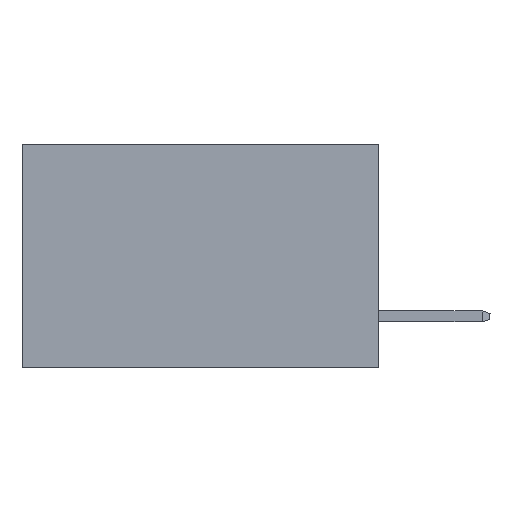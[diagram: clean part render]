
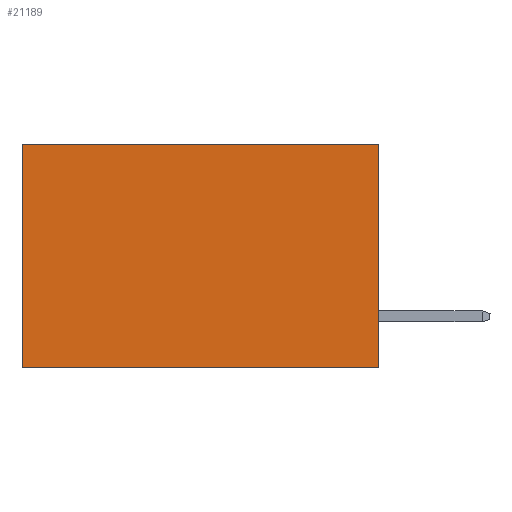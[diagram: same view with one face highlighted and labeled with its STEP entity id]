
A CAD part, left-side view. The second image highlights one B-rep face of the part: STEP entity #21189.
In plain terms, the highlighted planar face has unit normal (-1, 0, 0).
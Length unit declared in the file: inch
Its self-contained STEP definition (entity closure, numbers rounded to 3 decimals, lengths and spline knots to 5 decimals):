
#271 = DIRECTION ( 'NONE',  ( 0., 1., 0. ) ) ;
#390 = VECTOR ( 'NONE', #9604, 39.37008 ) ;
#517 = CARTESIAN_POINT ( 'NONE',  ( 0.277, 0., 0. ) ) ;
#1179 = LINE ( 'NONE', #7060, #390 ) ;
#1971 = VERTEX_POINT ( 'NONE', #30836 ) ;
#2939 = EDGE_LOOP ( 'NONE', ( #24589, #30960, #20420, #14679 ) ) ;
#3056 = VECTOR ( 'NONE', #11141, 39.37008 ) ;
#5113 = VERTEX_POINT ( 'NONE', #18928 ) ;
#5635 = DIRECTION ( 'NONE',  ( 0., 1., 0. ) ) ;
#7022 = LINE ( 'NONE', #517, #26850 ) ;
#7060 = CARTESIAN_POINT ( 'NONE',  ( 0.277, 0.59, -0.37 ) ) ;
#7666 = VERTEX_POINT ( 'NONE', #28542 ) ;
#7753 = DIRECTION ( 'NONE',  ( 1., 0., 0. ) ) ;
#7942 = CARTESIAN_POINT ( 'NONE',  ( 0.277, 0., -0.37 ) ) ;
#8642 = CARTESIAN_POINT ( 'NONE',  ( 0.277, 0., -0.37 ) ) ;
#9604 = DIRECTION ( 'NONE',  ( 0., 0., -1. ) ) ;
#11141 = DIRECTION ( 'NONE',  ( 0., 0., -1. ) ) ;
#11484 = VERTEX_POINT ( 'NONE', #25428 ) ;
#11711 = VECTOR ( 'NONE', #271, 39.37008 ) ;
#14679 = ORIENTED_EDGE ( 'NONE', *, *, #19999, .T. ) ;
#16407 = LINE ( 'NONE', #8642, #3056 ) ;
#18311 = LINE ( 'NONE', #7942, #11711 ) ;
#18928 = CARTESIAN_POINT ( 'NONE',  ( 0.277, 0.59, 0. ) ) ;
#19687 = EDGE_CURVE ( 'NONE', #7666, #11484, #16407, .T. ) ;
#19999 = EDGE_CURVE ( 'NONE', #7666, #5113, #7022, .T. ) ;
#20160 = PLANE ( 'NONE',  #29197 ) ;
#20420 = ORIENTED_EDGE ( 'NONE', *, *, #19687, .F. ) ;
#21189 = ADVANCED_FACE ( 'NONE', ( #27519 ), #20160, .F. ) ;
#24589 = ORIENTED_EDGE ( 'NONE', *, *, #27052, .T. ) ;
#25157 = DIRECTION ( 'NONE',  ( 0., 0., -1. ) ) ;
#25428 = CARTESIAN_POINT ( 'NONE',  ( 0.277, 0., -0.37 ) ) ;
#26850 = VECTOR ( 'NONE', #5635, 39.37008 ) ;
#27052 = EDGE_CURVE ( 'NONE', #5113, #1971, #1179, .T. ) ;
#27519 = FACE_OUTER_BOUND ( 'NONE', #2939, .T. ) ;
#28542 = CARTESIAN_POINT ( 'NONE',  ( 0.277, 0., 0. ) ) ;
#29197 = AXIS2_PLACEMENT_3D ( 'NONE', #29906, #7753, #25157 ) ;
#29543 = EDGE_CURVE ( 'NONE', #11484, #1971, #18311, .T. ) ;
#29906 = CARTESIAN_POINT ( 'NONE',  ( 0.277, 0., -0.37 ) ) ;
#30836 = CARTESIAN_POINT ( 'NONE',  ( 0.277, 0.59, -0.37 ) ) ;
#30960 = ORIENTED_EDGE ( 'NONE', *, *, #29543, .F. ) ;
